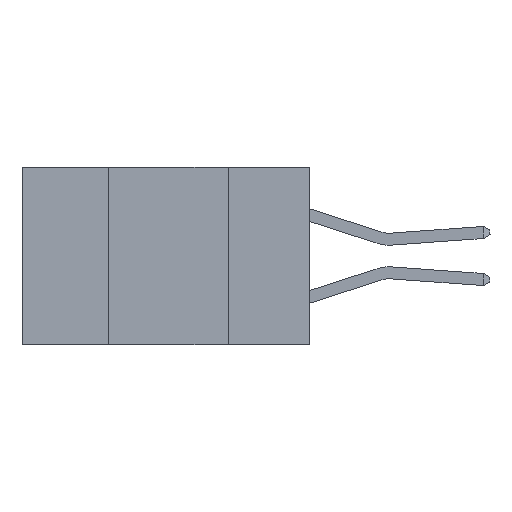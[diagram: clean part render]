
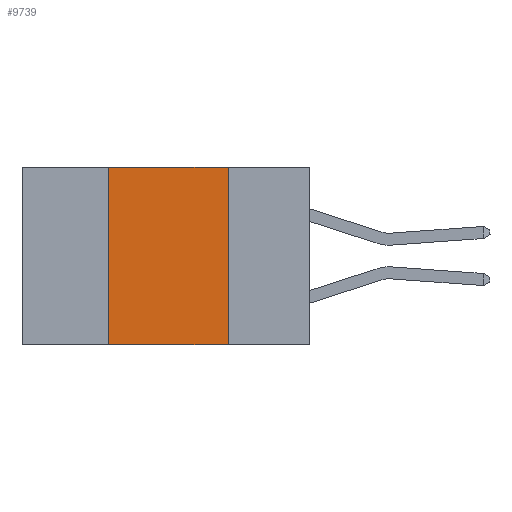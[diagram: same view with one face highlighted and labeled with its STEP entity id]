
A CAD part, left-side view. The second image highlights one B-rep face of the part: STEP entity #9739.
In plain terms, the highlighted planar face has unit normal (-1, 0, 0).
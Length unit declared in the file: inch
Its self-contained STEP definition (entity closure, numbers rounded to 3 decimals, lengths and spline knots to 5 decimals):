
#452 = CARTESIAN_POINT ( 'NONE',  ( 0., 0.17, 0. ) ) ;
#851 = VECTOR ( 'NONE', #11740, 39.37008 ) ;
#951 = DIRECTION ( 'NONE',  ( 0., 0., 1. ) ) ;
#1440 = CARTESIAN_POINT ( 'NONE',  ( 0., 0.42, 0. ) ) ;
#1951 = CARTESIAN_POINT ( 'NONE',  ( 0., 0.42, -0.37 ) ) ;
#2448 = VERTEX_POINT ( 'NONE', #3291 ) ;
#2522 = VERTEX_POINT ( 'NONE', #452 ) ;
#2806 = LINE ( 'NONE', #1951, #11140 ) ;
#3291 = CARTESIAN_POINT ( 'NONE',  ( 0., 0.42, -0.37 ) ) ;
#3837 = FACE_OUTER_BOUND ( 'NONE', #7891, .T. ) ;
#3900 = DIRECTION ( 'NONE',  ( 1., 0., 0. ) ) ;
#4218 = VERTEX_POINT ( 'NONE', #1440 ) ;
#4765 = CARTESIAN_POINT ( 'NONE',  ( 0., 0.6, 0. ) ) ;
#5046 = CARTESIAN_POINT ( 'NONE',  ( 0., 0.17, -0.37 ) ) ;
#5246 = EDGE_CURVE ( 'NONE', #4218, #2522, #12672, .T. ) ;
#5304 = LINE ( 'NONE', #5046, #10276 ) ;
#5538 = CARTESIAN_POINT ( 'NONE',  ( 0., 0.17, -0.37 ) ) ;
#5700 = CARTESIAN_POINT ( 'NONE',  ( 0., 0.6, -0.37 ) ) ;
#6750 = EDGE_CURVE ( 'NONE', #2522, #9988, #5304, .T. ) ;
#7179 = AXIS2_PLACEMENT_3D ( 'NONE', #4765, #3900, #8768 ) ;
#7853 = PLANE ( 'NONE',  #7179 ) ;
#7891 = EDGE_LOOP ( 'NONE', ( #11878, #8444, #9417, #9918 ) ) ;
#8444 = ORIENTED_EDGE ( 'NONE', *, *, #5246, .F. ) ;
#8708 = EDGE_CURVE ( 'NONE', #2448, #4218, #2806, .T. ) ;
#8768 = DIRECTION ( 'NONE',  ( 0., 0., -1. ) ) ;
#9008 = EDGE_CURVE ( 'NONE', #2448, #9988, #10747, .T. ) ;
#9417 = ORIENTED_EDGE ( 'NONE', *, *, #8708, .F. ) ;
#9639 = CARTESIAN_POINT ( 'NONE',  ( 0., 0.6, 0. ) ) ;
#9708 = DIRECTION ( 'NONE',  ( 0., -1., 0. ) ) ;
#9739 = ADVANCED_FACE ( 'NONE', ( #3837 ), #7853, .F. ) ;
#9918 = ORIENTED_EDGE ( 'NONE', *, *, #9008, .T. ) ;
#9988 = VERTEX_POINT ( 'NONE', #5538 ) ;
#10276 = VECTOR ( 'NONE', #11274, 39.37008 ) ;
#10747 = LINE ( 'NONE', #5700, #851 ) ;
#10883 = VECTOR ( 'NONE', #9708, 39.37008 ) ;
#11140 = VECTOR ( 'NONE', #951, 39.37008 ) ;
#11274 = DIRECTION ( 'NONE',  ( 0., 0., -1. ) ) ;
#11740 = DIRECTION ( 'NONE',  ( 0., -1., 0. ) ) ;
#11878 = ORIENTED_EDGE ( 'NONE', *, *, #6750, .F. ) ;
#12672 = LINE ( 'NONE', #9639, #10883 ) ;
